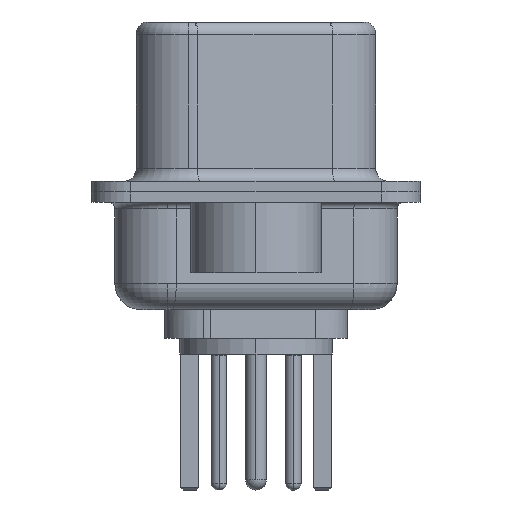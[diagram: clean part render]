
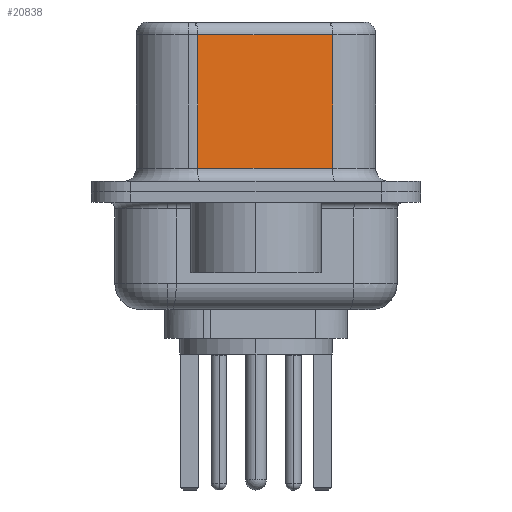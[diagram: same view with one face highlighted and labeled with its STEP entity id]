
A CAD part, left-side view. The second image highlights one B-rep face of the part: STEP entity #20838.
In plain terms, the highlighted planar face has unit normal (-0.985, -0.174, 0).
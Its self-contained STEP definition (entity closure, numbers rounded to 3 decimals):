
#62 = CARTESIAN_POINT ( 'NONE',  ( 3.67, 2.233, 0.9 ) ) ;
#90 = DIRECTION ( 'NONE',  ( 0., 0., -1. ) ) ;
#299 = CARTESIAN_POINT ( 'NONE',  ( 4.58, -2.927, 6.52 ) ) ;
#701 = LINE ( 'NONE', #18336, #23570 ) ;
#757 = DIRECTION ( 'NONE',  ( -0.174, 0.985, 0. ) ) ;
#1201 = LINE ( 'NONE', #9910, #12356 ) ;
#1537 = AXIS2_PLACEMENT_3D ( 'NONE', #299, #2510, #18122 ) ;
#1872 = EDGE_CURVE ( 'NONE', #16838, #18734, #11064, .T. ) ;
#2510 = DIRECTION ( 'NONE',  ( 0.985, 0.174, 0. ) ) ;
#3831 = CARTESIAN_POINT ( 'NONE',  ( 4.58, -2.927, 0.9 ) ) ;
#3910 = EDGE_CURVE ( 'NONE', #16838, #23762, #1201, .T. ) ;
#5023 = DIRECTION ( 'NONE',  ( 0., 0., -1. ) ) ;
#7432 = ORIENTED_EDGE ( 'NONE', *, *, #26926, .T. ) ;
#9858 = CARTESIAN_POINT ( 'NONE',  ( 4.58, -2.927, 0.9 ) ) ;
#9910 = CARTESIAN_POINT ( 'NONE',  ( 4.58, -2.927, 6.52 ) ) ;
#11064 = LINE ( 'NONE', #17305, #27872 ) ;
#11807 = CARTESIAN_POINT ( 'NONE',  ( 4.58, -2.927, 6.02 ) ) ;
#12356 = VECTOR ( 'NONE', #90, 1000. ) ;
#14377 = EDGE_CURVE ( 'NONE', #16092, #23762, #17058, .T. ) ;
#15311 = PLANE ( 'NONE',  #1537 ) ;
#16092 = VERTEX_POINT ( 'NONE', #62 ) ;
#16112 = ORIENTED_EDGE ( 'NONE', *, *, #14377, .T. ) ;
#16838 = VERTEX_POINT ( 'NONE', #11807 ) ;
#17058 = LINE ( 'NONE', #3831, #17749 ) ;
#17216 = DIRECTION ( 'NONE',  ( 0.174, -0.985, 0. ) ) ;
#17305 = CARTESIAN_POINT ( 'NONE',  ( 4.58, -2.927, 6.02 ) ) ;
#17749 = VECTOR ( 'NONE', #17216, 1000. ) ;
#17990 = FACE_OUTER_BOUND ( 'NONE', #20319, .T. ) ;
#18122 = DIRECTION ( 'NONE',  ( -0.174, 0.985, 0. ) ) ;
#18336 = CARTESIAN_POINT ( 'NONE',  ( 3.67, 2.233, 6.52 ) ) ;
#18734 = VERTEX_POINT ( 'NONE', #27025 ) ;
#19373 = ORIENTED_EDGE ( 'NONE', *, *, #3910, .F. ) ;
#20319 = EDGE_LOOP ( 'NONE', ( #19373, #26429, #7432, #16112 ) ) ;
#20838 = ADVANCED_FACE ( 'NONE', ( #17990 ), #15311, .F. ) ;
#23570 = VECTOR ( 'NONE', #5023, 1000. ) ;
#23762 = VERTEX_POINT ( 'NONE', #9858 ) ;
#26429 = ORIENTED_EDGE ( 'NONE', *, *, #1872, .T. ) ;
#26926 = EDGE_CURVE ( 'NONE', #18734, #16092, #701, .T. ) ;
#27025 = CARTESIAN_POINT ( 'NONE',  ( 3.67, 2.233, 6.02 ) ) ;
#27872 = VECTOR ( 'NONE', #757, 1000. ) ;
